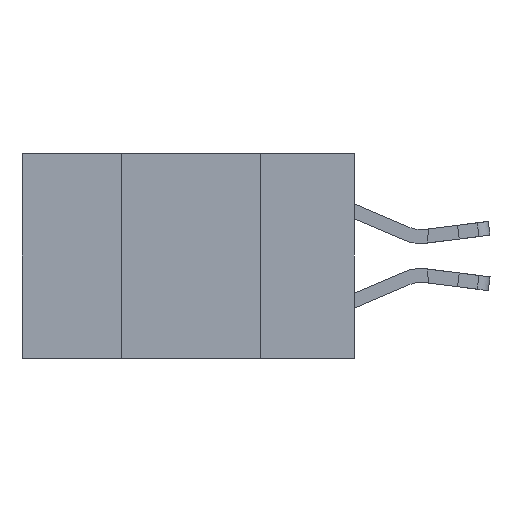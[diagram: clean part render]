
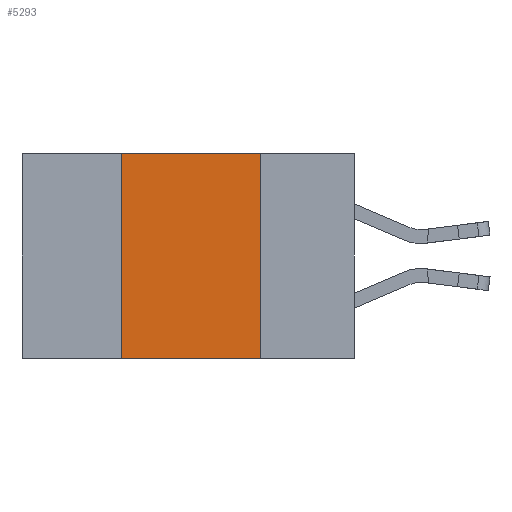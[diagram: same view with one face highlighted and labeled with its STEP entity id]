
A CAD part, left-side view. The second image highlights one B-rep face of the part: STEP entity #5293.
In plain terms, the highlighted planar face has unit normal (-1, 0, 0).
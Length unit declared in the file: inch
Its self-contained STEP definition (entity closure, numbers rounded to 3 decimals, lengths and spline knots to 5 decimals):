
#345 = ORIENTED_EDGE ( 'NONE', *, *, #19189, .F. ) ;
#511 = ORIENTED_EDGE ( 'NONE', *, *, #14937, .F. ) ;
#562 = ORIENTED_EDGE ( 'NONE', *, *, #11733, .T. ) ;
#1813 = ORIENTED_EDGE ( 'NONE', *, *, #7072, .F. ) ;
#2082 = VECTOR ( 'NONE', #18684, 39.37008 ) ;
#2544 = CARTESIAN_POINT ( 'NONE',  ( 0., 0.42, -0.37 ) ) ;
#3621 = CARTESIAN_POINT ( 'NONE',  ( 0., 0.17, -0.37 ) ) ;
#3828 = CARTESIAN_POINT ( 'NONE',  ( 0., 0.6, 0. ) ) ;
#4237 = VECTOR ( 'NONE', #20726, 39.37008 ) ;
#5293 = ADVANCED_FACE ( 'NONE', ( #12902 ), #7179, .F. ) ;
#6517 = LINE ( 'NONE', #16984, #2082 ) ;
#7072 = EDGE_CURVE ( 'NONE', #12229, #16071, #6517, .T. ) ;
#7179 = PLANE ( 'NONE',  #13857 ) ;
#7527 = CARTESIAN_POINT ( 'NONE',  ( 0., 0.42, 0. ) ) ;
#8712 = LINE ( 'NONE', #19110, #4237 ) ;
#8877 = DIRECTION ( 'NONE',  ( 0., 0., -1. ) ) ;
#9278 = EDGE_LOOP ( 'NONE', ( #1813, #345, #511, #562 ) ) ;
#10395 = LINE ( 'NONE', #12509, #13812 ) ;
#11236 = VERTEX_POINT ( 'NONE', #7527 ) ;
#11733 = EDGE_CURVE ( 'NONE', #17248, #16071, #10395, .T. ) ;
#12229 = VERTEX_POINT ( 'NONE', #13919 ) ;
#12509 = CARTESIAN_POINT ( 'NONE',  ( 0., 0.6, -0.37 ) ) ;
#12902 = FACE_OUTER_BOUND ( 'NONE', #9278, .T. ) ;
#13812 = VECTOR ( 'NONE', #19065, 39.37008 ) ;
#13857 = AXIS2_PLACEMENT_3D ( 'NONE', #3828, #18757, #8877 ) ;
#13919 = CARTESIAN_POINT ( 'NONE',  ( 0., 0.17, 0. ) ) ;
#14937 = EDGE_CURVE ( 'NONE', #17248, #11236, #15662, .T. ) ;
#15162 = VECTOR ( 'NONE', #15888, 39.37008 ) ;
#15662 = LINE ( 'NONE', #2544, #15162 ) ;
#15888 = DIRECTION ( 'NONE',  ( 0., 0., 1. ) ) ;
#16071 = VERTEX_POINT ( 'NONE', #3621 ) ;
#16984 = CARTESIAN_POINT ( 'NONE',  ( 0., 0.17, -0.37 ) ) ;
#17248 = VERTEX_POINT ( 'NONE', #21342 ) ;
#18684 = DIRECTION ( 'NONE',  ( 0., 0., -1. ) ) ;
#18757 = DIRECTION ( 'NONE',  ( 1., 0., 0. ) ) ;
#19065 = DIRECTION ( 'NONE',  ( 0., -1., 0. ) ) ;
#19110 = CARTESIAN_POINT ( 'NONE',  ( 0., 0.6, 0. ) ) ;
#19189 = EDGE_CURVE ( 'NONE', #11236, #12229, #8712, .T. ) ;
#20726 = DIRECTION ( 'NONE',  ( 0., -1., 0. ) ) ;
#21342 = CARTESIAN_POINT ( 'NONE',  ( 0., 0.42, -0.37 ) ) ;
